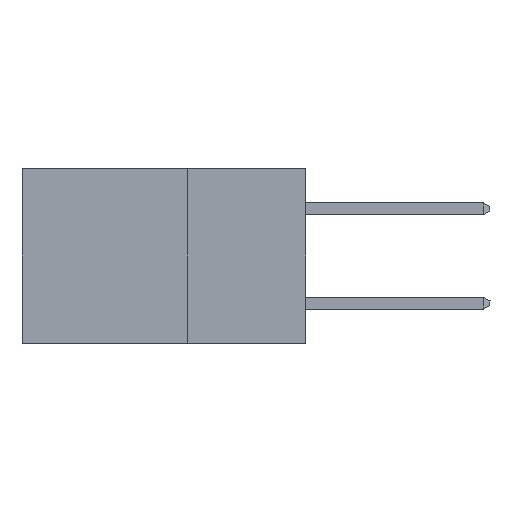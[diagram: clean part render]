
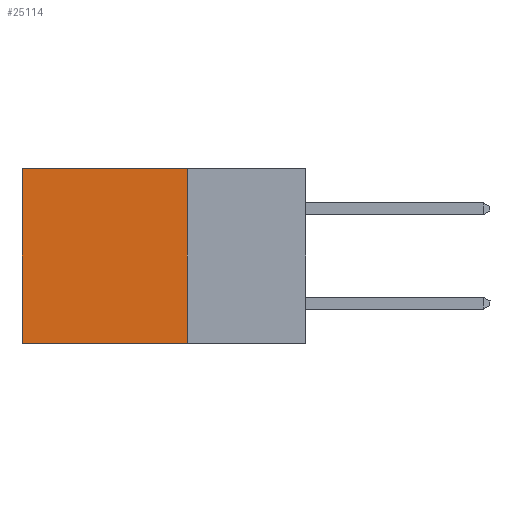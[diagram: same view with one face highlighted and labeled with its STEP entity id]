
A CAD part, left-side view. The second image highlights one B-rep face of the part: STEP entity #25114.
In plain terms, the highlighted planar face has unit normal (-1, 0, 0).
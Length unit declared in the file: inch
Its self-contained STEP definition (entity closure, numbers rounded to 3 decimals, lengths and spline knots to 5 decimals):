
#1911 = CARTESIAN_POINT ( 'NONE',  ( 0.298, 0.25, 0. ) ) ;
#3296 = CARTESIAN_POINT ( 'NONE',  ( 0.298, 0.6, -0.37 ) ) ;
#3357 = EDGE_CURVE ( 'NONE', #26791, #25772, #24822, .T. ) ;
#4048 = VECTOR ( 'NONE', #4666, 39.37008 ) ;
#4129 = CARTESIAN_POINT ( 'NONE',  ( 0.298, 0.6, 0. ) ) ;
#4666 = DIRECTION ( 'NONE',  ( 0., 1., 0. ) ) ;
#5436 = EDGE_CURVE ( 'NONE', #7094, #25772, #7412, .T. ) ;
#6075 = LINE ( 'NONE', #10768, #19431 ) ;
#6493 = CARTESIAN_POINT ( 'NONE',  ( 0.298, 0.25, 0. ) ) ;
#6746 = VERTEX_POINT ( 'NONE', #14964 ) ;
#7094 = VERTEX_POINT ( 'NONE', #7580 ) ;
#7412 = LINE ( 'NONE', #23473, #4048 ) ;
#7580 = CARTESIAN_POINT ( 'NONE',  ( 0.298, 0.25, -0.37 ) ) ;
#10768 = CARTESIAN_POINT ( 'NONE',  ( 0.298, 0.25, 0. ) ) ;
#11705 = ORIENTED_EDGE ( 'NONE', *, *, #29284, .F. ) ;
#12042 = ORIENTED_EDGE ( 'NONE', *, *, #3357, .T. ) ;
#12787 = AXIS2_PLACEMENT_3D ( 'NONE', #1911, #18456, #23565 ) ;
#14964 = CARTESIAN_POINT ( 'NONE',  ( 0.298, 0.25, 0. ) ) ;
#16234 = DIRECTION ( 'NONE',  ( 0., 1., 0. ) ) ;
#18012 = VECTOR ( 'NONE', #16234, 39.37008 ) ;
#18456 = DIRECTION ( 'NONE',  ( 1., 0., 0. ) ) ;
#19297 = FACE_OUTER_BOUND ( 'NONE', #29642, .T. ) ;
#19431 = VECTOR ( 'NONE', #20621, 39.37008 ) ;
#20504 = ORIENTED_EDGE ( 'NONE', *, *, #30209, .T. ) ;
#20621 = DIRECTION ( 'NONE',  ( 0., 0., -1. ) ) ;
#21082 = PLANE ( 'NONE',  #12787 ) ;
#23149 = CARTESIAN_POINT ( 'NONE',  ( 0.298, 0.6, 0. ) ) ;
#23473 = CARTESIAN_POINT ( 'NONE',  ( 0.298, 0.25, -0.37 ) ) ;
#23565 = DIRECTION ( 'NONE',  ( 0., 0., -1. ) ) ;
#24452 = VECTOR ( 'NONE', #25554, 39.37008 ) ;
#24822 = LINE ( 'NONE', #23149, #24452 ) ;
#25114 = ADVANCED_FACE ( 'NONE', ( #19297 ), #21082, .F. ) ;
#25554 = DIRECTION ( 'NONE',  ( 0., 0., -1. ) ) ;
#25772 = VERTEX_POINT ( 'NONE', #3296 ) ;
#26791 = VERTEX_POINT ( 'NONE', #4129 ) ;
#28400 = ORIENTED_EDGE ( 'NONE', *, *, #5436, .F. ) ;
#29284 = EDGE_CURVE ( 'NONE', #6746, #7094, #6075, .T. ) ;
#29631 = LINE ( 'NONE', #6493, #18012 ) ;
#29642 = EDGE_LOOP ( 'NONE', ( #12042, #28400, #11705, #20504 ) ) ;
#30209 = EDGE_CURVE ( 'NONE', #6746, #26791, #29631, .T. ) ;
